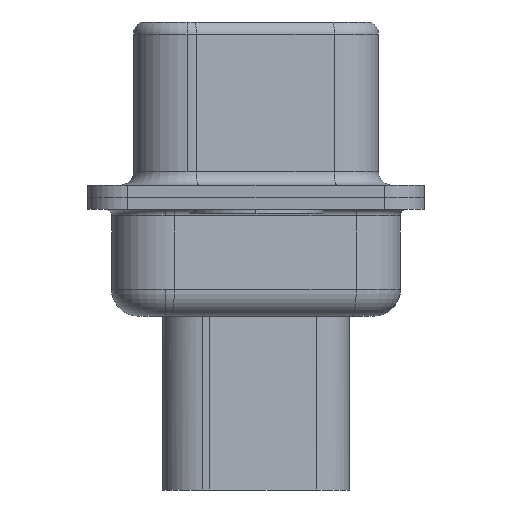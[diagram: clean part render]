
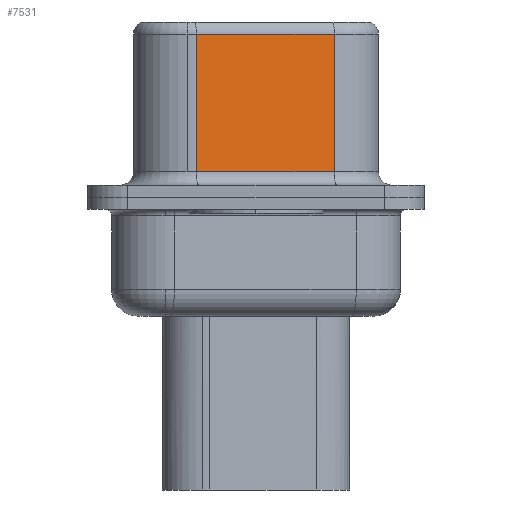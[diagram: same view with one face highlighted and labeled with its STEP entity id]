
A CAD part, left-side view. The second image highlights one B-rep face of the part: STEP entity #7531.
In plain terms, the highlighted planar face has unit normal (-0.985, -0.174, 0).
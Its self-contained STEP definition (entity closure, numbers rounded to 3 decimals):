
#489 = VERTEX_POINT ( 'NONE', #6351 ) ;
#791 = VERTEX_POINT ( 'NONE', #9374 ) ;
#820 = VERTEX_POINT ( 'NONE', #10054 ) ;
#955 = ORIENTED_EDGE ( 'NONE', *, *, #9513, .T. ) ;
#1388 = CARTESIAN_POINT ( 'NONE',  ( 4.575, -2.927, 0.95 ) ) ;
#1787 = EDGE_CURVE ( 'NONE', #5112, #489, #5215, .T. ) ;
#2783 = DIRECTION ( 'NONE',  ( -0.174, 0.985, 0. ) ) ;
#2947 = LINE ( 'NONE', #8340, #7257 ) ;
#3451 = VECTOR ( 'NONE', #9981, 1000. ) ;
#3574 = PLANE ( 'NONE',  #5080 ) ;
#4401 = EDGE_LOOP ( 'NONE', ( #7327, #10373, #955, #6693 ) ) ;
#5080 = AXIS2_PLACEMENT_3D ( 'NONE', #6772, #9958, #2783 ) ;
#5102 = VECTOR ( 'NONE', #10205, 1000. ) ;
#5112 = VERTEX_POINT ( 'NONE', #10048 ) ;
#5215 = LINE ( 'NONE', #9044, #3451 ) ;
#5602 = VECTOR ( 'NONE', #6648, 1000. ) ;
#6351 = CARTESIAN_POINT ( 'NONE',  ( 4.575, -2.927, 0.95 ) ) ;
#6648 = DIRECTION ( 'NONE',  ( 0., 0., -1. ) ) ;
#6693 = ORIENTED_EDGE ( 'NONE', *, *, #9894, .T. ) ;
#6772 = CARTESIAN_POINT ( 'NONE',  ( 4.575, -2.927, 6.55 ) ) ;
#6933 = FACE_OUTER_BOUND ( 'NONE', #4401, .T. ) ;
#7257 = VECTOR ( 'NONE', #9276, 1000. ) ;
#7327 = ORIENTED_EDGE ( 'NONE', *, *, #1787, .F. ) ;
#7404 = EDGE_CURVE ( 'NONE', #5112, #820, #2947, .T. ) ;
#7531 = ADVANCED_FACE ( 'NONE', ( #6933 ), #3574, .F. ) ;
#8340 = CARTESIAN_POINT ( 'NONE',  ( 4.575, -2.927, 6.1 ) ) ;
#8584 = LINE ( 'NONE', #1388, #5102 ) ;
#8905 = CARTESIAN_POINT ( 'NONE',  ( 3.665, 2.233, 6.55 ) ) ;
#9003 = LINE ( 'NONE', #8905, #5602 ) ;
#9044 = CARTESIAN_POINT ( 'NONE',  ( 4.575, -2.927, 6.55 ) ) ;
#9276 = DIRECTION ( 'NONE',  ( -0.174, 0.985, 0. ) ) ;
#9374 = CARTESIAN_POINT ( 'NONE',  ( 3.665, 2.233, 0.95 ) ) ;
#9513 = EDGE_CURVE ( 'NONE', #820, #791, #9003, .T. ) ;
#9894 = EDGE_CURVE ( 'NONE', #791, #489, #8584, .T. ) ;
#9958 = DIRECTION ( 'NONE',  ( 0.985, 0.174, 0. ) ) ;
#9981 = DIRECTION ( 'NONE',  ( 0., 0., -1. ) ) ;
#10048 = CARTESIAN_POINT ( 'NONE',  ( 4.575, -2.927, 6.1 ) ) ;
#10054 = CARTESIAN_POINT ( 'NONE',  ( 3.665, 2.233, 6.1 ) ) ;
#10205 = DIRECTION ( 'NONE',  ( 0.174, -0.985, 0. ) ) ;
#10373 = ORIENTED_EDGE ( 'NONE', *, *, #7404, .T. ) ;
